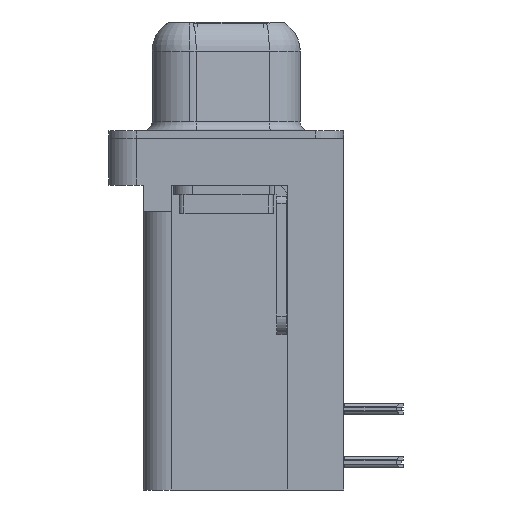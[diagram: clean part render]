
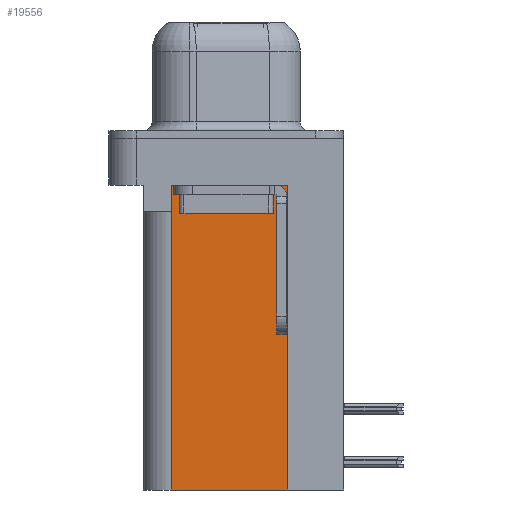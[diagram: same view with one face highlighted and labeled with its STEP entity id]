
A CAD part, left-side view. The second image highlights one B-rep face of the part: STEP entity #19556.
In plain terms, the highlighted planar face has unit normal (-1, 0, 0).
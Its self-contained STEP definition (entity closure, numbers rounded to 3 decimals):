
#1093 = VECTOR ( 'NONE', #5408, 1000. ) ;
#1562 = VECTOR ( 'NONE', #33759, 1000. ) ;
#1947 = LINE ( 'NONE', #24841, #1093 ) ;
#3418 = CARTESIAN_POINT ( 'NONE',  ( 3.79, -3.295, -18.76 ) ) ;
#4320 = VECTOR ( 'NONE', #11646, 1000. ) ;
#4988 = CARTESIAN_POINT ( 'NONE',  ( 3.79, 2.925, -18.76 ) ) ;
#5408 = DIRECTION ( 'NONE',  ( 0., 1., 0. ) ) ;
#5912 = CARTESIAN_POINT ( 'NONE',  ( 3.79, 2.895, -3.9 ) ) ;
#7797 = VECTOR ( 'NONE', #17667, 1000. ) ;
#7813 = VERTEX_POINT ( 'NONE', #4988 ) ;
#8402 = EDGE_CURVE ( 'NONE', #13782, #11152, #10484, .T. ) ;
#9826 = ORIENTED_EDGE ( 'NONE', *, *, #30102, .F. ) ;
#10007 = LINE ( 'NONE', #30994, #1562 ) ;
#10156 = DIRECTION ( 'NONE',  ( 0., 1., 0. ) ) ;
#10435 = VERTEX_POINT ( 'NONE', #10737 ) ;
#10484 = LINE ( 'NONE', #5912, #18677 ) ;
#10737 = CARTESIAN_POINT ( 'NONE',  ( 3.79, -3.295, -18.76 ) ) ;
#11152 = VERTEX_POINT ( 'NONE', #14073 ) ;
#11646 = DIRECTION ( 'NONE',  ( 0., 1., 0. ) ) ;
#11778 = LINE ( 'NONE', #25425, #4320 ) ;
#12139 = EDGE_LOOP ( 'NONE', ( #24749, #34592, #32863, #30834, #9826, #27914 ) ) ;
#13105 = CARTESIAN_POINT ( 'NONE',  ( 3.79, -3.295, -2.5 ) ) ;
#13782 = VERTEX_POINT ( 'NONE', #31036 ) ;
#14073 = CARTESIAN_POINT ( 'NONE',  ( 3.79, 2.895, -3.9 ) ) ;
#15125 = LINE ( 'NONE', #31419, #7797 ) ;
#16352 = VERTEX_POINT ( 'NONE', #25632 ) ;
#17667 = DIRECTION ( 'NONE',  ( 0., 0., 1. ) ) ;
#17976 = FACE_OUTER_BOUND ( 'NONE', #12139, .T. ) ;
#18677 = VECTOR ( 'NONE', #25333, 1000. ) ;
#19556 = ADVANCED_FACE ( 'NONE', ( #17976 ), #21176, .F. ) ;
#21176 = PLANE ( 'NONE',  #30224 ) ;
#22751 = EDGE_CURVE ( 'NONE', #10435, #24276, #10007, .T. ) ;
#22931 = DIRECTION ( 'NONE',  ( 0., 1., 0. ) ) ;
#23950 = CARTESIAN_POINT ( 'NONE',  ( 3.79, -3.295, -18.76 ) ) ;
#23980 = LINE ( 'NONE', #3418, #31293 ) ;
#24276 = VERTEX_POINT ( 'NONE', #13105 ) ;
#24412 = EDGE_CURVE ( 'NONE', #24276, #13782, #1947, .T. ) ;
#24749 = ORIENTED_EDGE ( 'NONE', *, *, #24412, .T. ) ;
#24841 = CARTESIAN_POINT ( 'NONE',  ( 3.79, -3.295, -2.5 ) ) ;
#25333 = DIRECTION ( 'NONE',  ( 0., 0., -1. ) ) ;
#25425 = CARTESIAN_POINT ( 'NONE',  ( 3.79, 0., -3.9 ) ) ;
#25632 = CARTESIAN_POINT ( 'NONE',  ( 3.79, 2.925, -3.9 ) ) ;
#26693 = DIRECTION ( 'NONE',  ( 1., 0., 0. ) ) ;
#27914 = ORIENTED_EDGE ( 'NONE', *, *, #22751, .T. ) ;
#30102 = EDGE_CURVE ( 'NONE', #10435, #7813, #23980, .T. ) ;
#30224 = AXIS2_PLACEMENT_3D ( 'NONE', #23950, #26693, #10156 ) ;
#30834 = ORIENTED_EDGE ( 'NONE', *, *, #33114, .F. ) ;
#30994 = CARTESIAN_POINT ( 'NONE',  ( 3.79, -3.295, -18.76 ) ) ;
#31036 = CARTESIAN_POINT ( 'NONE',  ( 3.79, 2.895, -2.5 ) ) ;
#31293 = VECTOR ( 'NONE', #22931, 1000. ) ;
#31419 = CARTESIAN_POINT ( 'NONE',  ( 3.79, 2.925, -18.76 ) ) ;
#32022 = EDGE_CURVE ( 'NONE', #11152, #16352, #11778, .T. ) ;
#32863 = ORIENTED_EDGE ( 'NONE', *, *, #32022, .T. ) ;
#33114 = EDGE_CURVE ( 'NONE', #7813, #16352, #15125, .T. ) ;
#33759 = DIRECTION ( 'NONE',  ( 0., 0., 1. ) ) ;
#34592 = ORIENTED_EDGE ( 'NONE', *, *, #8402, .T. ) ;
